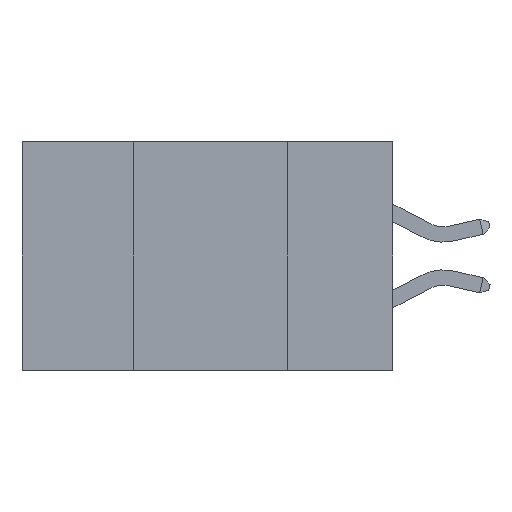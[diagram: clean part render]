
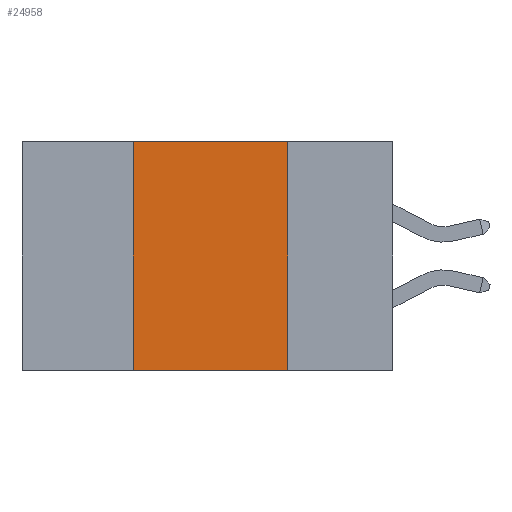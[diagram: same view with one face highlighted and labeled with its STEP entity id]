
A CAD part, left-side view. The second image highlights one B-rep face of the part: STEP entity #24958.
In plain terms, the highlighted planar face has unit normal (-1, 0, 0).
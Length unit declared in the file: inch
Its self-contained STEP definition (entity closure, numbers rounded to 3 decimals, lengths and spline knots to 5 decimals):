
#1498 = VECTOR ( 'NONE', #3025, 39.37008 ) ;
#2523 = VECTOR ( 'NONE', #28927, 39.37008 ) ;
#3025 = DIRECTION ( 'NONE',  ( 0., 0., -1. ) ) ;
#3972 = DIRECTION ( 'NONE',  ( 0., -1., 0. ) ) ;
#4098 = LINE ( 'NONE', #26873, #2523 ) ;
#6324 = VERTEX_POINT ( 'NONE', #13786 ) ;
#8107 = VECTOR ( 'NONE', #26227, 39.37008 ) ;
#8906 = DIRECTION ( 'NONE',  ( 0., 0., -1. ) ) ;
#9102 = DIRECTION ( 'NONE',  ( 1., 0., 0. ) ) ;
#9282 = CARTESIAN_POINT ( 'NONE',  ( 0., 0.6, 0. ) ) ;
#10745 = ORIENTED_EDGE ( 'NONE', *, *, #20198, .F. ) ;
#11510 = LINE ( 'NONE', #9282, #8107 ) ;
#11604 = EDGE_CURVE ( 'NONE', #11783, #24394, #11510, .T. ) ;
#11732 = PLANE ( 'NONE',  #26610 ) ;
#11783 = VERTEX_POINT ( 'NONE', #22147 ) ;
#13786 = CARTESIAN_POINT ( 'NONE',  ( 0., 0.17, -0.37 ) ) ;
#13836 = ORIENTED_EDGE ( 'NONE', *, *, #26858, .T. ) ;
#15403 = FACE_OUTER_BOUND ( 'NONE', #30350, .T. ) ;
#16017 = ORIENTED_EDGE ( 'NONE', *, *, #11604, .F. ) ;
#16164 = CARTESIAN_POINT ( 'NONE',  ( 0., 0.6, 0. ) ) ;
#16718 = CARTESIAN_POINT ( 'NONE',  ( 0., 0.17, 0. ) ) ;
#17966 = VECTOR ( 'NONE', #3972, 39.37008 ) ;
#18147 = LINE ( 'NONE', #24968, #1498 ) ;
#19110 = LINE ( 'NONE', #23658, #17966 ) ;
#20198 = EDGE_CURVE ( 'NONE', #24394, #6324, #18147, .T. ) ;
#21910 = EDGE_CURVE ( 'NONE', #22397, #11783, #4098, .T. ) ;
#22147 = CARTESIAN_POINT ( 'NONE',  ( 0., 0.42, 0. ) ) ;
#22397 = VERTEX_POINT ( 'NONE', #23570 ) ;
#23570 = CARTESIAN_POINT ( 'NONE',  ( 0., 0.42, -0.37 ) ) ;
#23658 = CARTESIAN_POINT ( 'NONE',  ( 0., 0.6, -0.37 ) ) ;
#24394 = VERTEX_POINT ( 'NONE', #16718 ) ;
#24958 = ADVANCED_FACE ( 'NONE', ( #15403 ), #11732, .F. ) ;
#24968 = CARTESIAN_POINT ( 'NONE',  ( 0., 0.17, 0. ) ) ;
#26227 = DIRECTION ( 'NONE',  ( 0., -1., 0. ) ) ;
#26610 = AXIS2_PLACEMENT_3D ( 'NONE', #16164, #9102, #8906 ) ;
#26858 = EDGE_CURVE ( 'NONE', #22397, #6324, #19110, .T. ) ;
#26873 = CARTESIAN_POINT ( 'NONE',  ( 0., 0.42, 0. ) ) ;
#28927 = DIRECTION ( 'NONE',  ( 0., 0., 1. ) ) ;
#30328 = ORIENTED_EDGE ( 'NONE', *, *, #21910, .F. ) ;
#30350 = EDGE_LOOP ( 'NONE', ( #10745, #16017, #30328, #13836 ) ) ;
